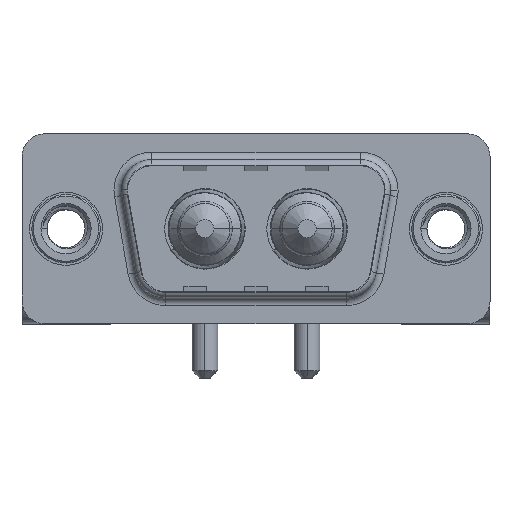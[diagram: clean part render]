
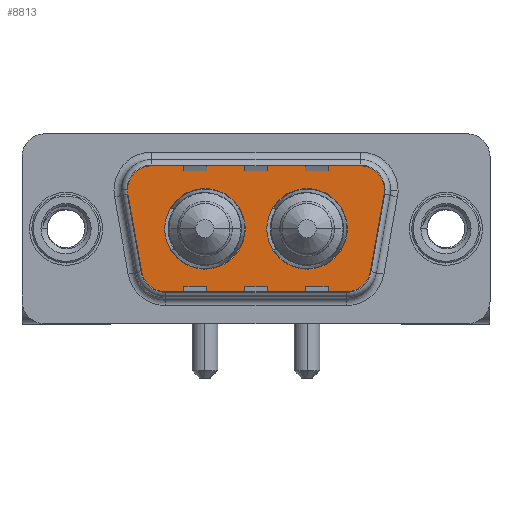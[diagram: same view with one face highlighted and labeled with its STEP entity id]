
A CAD part, top view. The second image highlights one B-rep face of the part: STEP entity #8813.
In plain terms, the highlighted planar face has unit normal (0, 0, 1).
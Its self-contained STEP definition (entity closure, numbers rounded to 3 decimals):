
#17 = LINE ( 'NONE', #8487, #10668 ) ;
#69 = VERTEX_POINT ( 'NONE', #1783 ) ;
#195 = VECTOR ( 'NONE', #10316, 1000. ) ;
#313 = ORIENTED_EDGE ( 'NONE', *, *, #13382, .T. ) ;
#531 = EDGE_CURVE ( 'NONE', #8651, #4644, #12006, .T. ) ;
#673 = AXIS2_PLACEMENT_3D ( 'NONE', #11711, #11919, #10384 ) ;
#860 = CARTESIAN_POINT ( 'NONE',  ( 15.86, 0., 0. ) ) ;
#886 = ORIENTED_EDGE ( 'NONE', *, *, #9757, .T. ) ;
#1145 = CIRCLE ( 'NONE', #2961, 2. ) ;
#1183 = CIRCLE ( 'NONE', #9352, 2.65 ) ;
#1215 = VERTEX_POINT ( 'NONE', #11139 ) ;
#1319 = ORIENTED_EDGE ( 'NONE', *, *, #2807, .F. ) ;
#1494 = AXIS2_PLACEMENT_3D ( 'NONE', #12614, #7407, #1807 ) ;
#1783 = CARTESIAN_POINT ( 'NONE',  ( 11.79, 0., 0. ) ) ;
#1807 = DIRECTION ( 'NONE',  ( 1., 0., 0. ) ) ;
#1871 = AXIS2_PLACEMENT_3D ( 'NONE', #4380, #8710, #12273 ) ;
#1963 = VECTOR ( 'NONE', #3189, 1000. ) ;
#1979 = DIRECTION ( 'NONE',  ( 0., 0., 1. ) ) ;
#2254 = EDGE_CURVE ( 'NONE', #3046, #11323, #12685, .T. ) ;
#2335 = EDGE_CURVE ( 'NONE', #69, #5789, #7602, .T. ) ;
#2347 = CARTESIAN_POINT ( 'NONE',  ( 19.564, 4.9, 0. ) ) ;
#2535 = ORIENTED_EDGE ( 'NONE', *, *, #11540, .F. ) ;
#2633 = DIRECTION ( 'NONE',  ( 0., 0., 1. ) ) ;
#2807 = EDGE_CURVE ( 'NONE', #4644, #8651, #10326, .T. ) ;
#2851 = FACE_BOUND ( 'NONE', #9070, .T. ) ;
#2918 = CARTESIAN_POINT ( 'NONE',  ( 18.541, -2.9, 0. ) ) ;
#2961 = AXIS2_PLACEMENT_3D ( 'NONE', #13447, #7103, #10376 ) ;
#3046 = VERTEX_POINT ( 'NONE', #2347 ) ;
#3189 = DIRECTION ( 'NONE',  ( 0.174, -0.985, 0. ) ) ;
#3738 = AXIS2_PLACEMENT_3D ( 'NONE', #860, #13870, #12666 ) ;
#3829 = EDGE_CURVE ( 'NONE', #12313, #10613, #10870, .T. ) ;
#3947 = CARTESIAN_POINT ( 'NONE',  ( 20.511, -3.247, 0. ) ) ;
#4380 = CARTESIAN_POINT ( 'NONE',  ( 19.564, 2.9, 0. ) ) ;
#4626 = CARTESIAN_POINT ( 'NONE',  ( 6.459, -4.9, 0. ) ) ;
#4630 = ORIENTED_EDGE ( 'NONE', *, *, #7220, .T. ) ;
#4644 = VERTEX_POINT ( 'NONE', #10782 ) ;
#4932 = DIRECTION ( 'NONE',  ( 1., 0., 0. ) ) ;
#4981 = VERTEX_POINT ( 'NONE', #11244 ) ;
#5092 = EDGE_LOOP ( 'NONE', ( #313, #8845, #9042, #886, #14020, #4630, #5809, #10586, #8516 ) ) ;
#5184 = FACE_BOUND ( 'NONE', #7694, .T. ) ;
#5206 = CIRCLE ( 'NONE', #673, 2. ) ;
#5745 = CARTESIAN_POINT ( 'NONE',  ( 6.459, -2.9, 0. ) ) ;
#5789 = VERTEX_POINT ( 'NONE', #12716 ) ;
#5809 = ORIENTED_EDGE ( 'NONE', *, *, #3829, .T. ) ;
#5972 = EDGE_CURVE ( 'NONE', #13334, #9483, #11846, .T. ) ;
#6006 = DIRECTION ( 'NONE',  ( 0., 0., 1. ) ) ;
#6139 = VERTEX_POINT ( 'NONE', #3947 ) ;
#6178 = AXIS2_PLACEMENT_3D ( 'NONE', #2918, #13797, #11588 ) ;
#7091 = EDGE_CURVE ( 'NONE', #4981, #1215, #13589, .T. ) ;
#7094 = AXIS2_PLACEMENT_3D ( 'NONE', #5745, #2633, #7872 ) ;
#7103 = DIRECTION ( 'NONE',  ( 0., 0., 1. ) ) ;
#7176 = FACE_OUTER_BOUND ( 'NONE', #5092, .T. ) ;
#7220 = EDGE_CURVE ( 'NONE', #11323, #12313, #5206, .T. ) ;
#7338 = DIRECTION ( 'NONE',  ( -1., 0., 0. ) ) ;
#7407 = DIRECTION ( 'NONE',  ( 0., 0., 1. ) ) ;
#7602 = CIRCLE ( 'NONE', #1494, 2.65 ) ;
#7645 = EDGE_CURVE ( 'NONE', #6139, #13334, #17, .T. ) ;
#7694 = EDGE_LOOP ( 'NONE', ( #7771, #2535 ) ) ;
#7771 = ORIENTED_EDGE ( 'NONE', *, *, #2335, .F. ) ;
#7872 = DIRECTION ( 'NONE',  ( -1., 0., 0. ) ) ;
#7877 = CIRCLE ( 'NONE', #13337, 2. ) ;
#8261 = ORIENTED_EDGE ( 'NONE', *, *, #531, .F. ) ;
#8487 = CARTESIAN_POINT ( 'NONE',  ( 21.534, 2.553, 0. ) ) ;
#8516 = ORIENTED_EDGE ( 'NONE', *, *, #7091, .T. ) ;
#8531 = CARTESIAN_POINT ( 'NONE',  ( 21.564, 2.9, 0. ) ) ;
#8651 = VERTEX_POINT ( 'NONE', #9173 ) ;
#8710 = DIRECTION ( 'NONE',  ( 0., 0., 1. ) ) ;
#8813 = ADVANCED_FACE ( 'NONE', ( #2851, #5184, #7176 ), #10455, .T. ) ;
#8845 = ORIENTED_EDGE ( 'NONE', *, *, #7645, .T. ) ;
#9038 = EDGE_CURVE ( 'NONE', #10613, #4981, #9348, .T. ) ;
#9042 = ORIENTED_EDGE ( 'NONE', *, *, #5972, .T. ) ;
#9070 = EDGE_LOOP ( 'NONE', ( #1319, #8261 ) ) ;
#9173 = CARTESIAN_POINT ( 'NONE',  ( 13.21, 0., 0. ) ) ;
#9348 = CIRCLE ( 'NONE', #7094, 2. ) ;
#9352 = AXIS2_PLACEMENT_3D ( 'NONE', #11413, #6006, #4932 ) ;
#9483 = VERTEX_POINT ( 'NONE', #8531 ) ;
#9757 = EDGE_CURVE ( 'NONE', #9483, #3046, #1145, .T. ) ;
#9802 = DIRECTION ( 'NONE',  ( 0., 0., 1. ) ) ;
#9943 = CARTESIAN_POINT ( 'NONE',  ( 15.86, 0., 0. ) ) ;
#10316 = DIRECTION ( 'NONE',  ( 1., 0., 0. ) ) ;
#10326 = CIRCLE ( 'NONE', #3738, 2.65 ) ;
#10371 = CARTESIAN_POINT ( 'NONE',  ( 21.534, 2.553, 0. ) ) ;
#10376 = DIRECTION ( 'NONE',  ( -1., 0., 0. ) ) ;
#10384 = DIRECTION ( 'NONE',  ( 1., 0., 0. ) ) ;
#10455 = PLANE ( 'NONE',  #6178 ) ;
#10586 = ORIENTED_EDGE ( 'NONE', *, *, #9038, .T. ) ;
#10613 = VERTEX_POINT ( 'NONE', #13670 ) ;
#10646 = DIRECTION ( 'NONE',  ( 1., 0., 0. ) ) ;
#10668 = VECTOR ( 'NONE', #13833, 1000. ) ;
#10776 = CARTESIAN_POINT ( 'NONE',  ( 5.436, 4.9, 0. ) ) ;
#10782 = CARTESIAN_POINT ( 'NONE',  ( 18.51, 0., 0. ) ) ;
#10870 = LINE ( 'NONE', #12941, #1963 ) ;
#10951 = DIRECTION ( 'NONE',  ( 1., 0., 0. ) ) ;
#11139 = CARTESIAN_POINT ( 'NONE',  ( 18.541, -4.9, 0. ) ) ;
#11244 = CARTESIAN_POINT ( 'NONE',  ( 6.459, -4.9, 0. ) ) ;
#11254 = VECTOR ( 'NONE', #7338, 1000. ) ;
#11323 = VERTEX_POINT ( 'NONE', #10776 ) ;
#11335 = AXIS2_PLACEMENT_3D ( 'NONE', #9943, #9802, #10951 ) ;
#11413 = CARTESIAN_POINT ( 'NONE',  ( 9.14, 0., 0. ) ) ;
#11540 = EDGE_CURVE ( 'NONE', #5789, #69, #1183, .T. ) ;
#11588 = DIRECTION ( 'NONE',  ( 1., 0., 0. ) ) ;
#11711 = CARTESIAN_POINT ( 'NONE',  ( 5.436, 2.9, 0. ) ) ;
#11714 = CARTESIAN_POINT ( 'NONE',  ( 18.541, -2.9, 0. ) ) ;
#11846 = CIRCLE ( 'NONE', #1871, 2. ) ;
#11919 = DIRECTION ( 'NONE',  ( 0., 0., 1. ) ) ;
#12006 = CIRCLE ( 'NONE', #11335, 2.65 ) ;
#12273 = DIRECTION ( 'NONE',  ( -1., 0., 0. ) ) ;
#12313 = VERTEX_POINT ( 'NONE', #13317 ) ;
#12614 = CARTESIAN_POINT ( 'NONE',  ( 9.14, 0., 0. ) ) ;
#12666 = DIRECTION ( 'NONE',  ( 1., 0., 0. ) ) ;
#12685 = LINE ( 'NONE', #13818, #11254 ) ;
#12716 = CARTESIAN_POINT ( 'NONE',  ( 6.49, 0., 0. ) ) ;
#12941 = CARTESIAN_POINT ( 'NONE',  ( 3.466, 2.553, 0. ) ) ;
#13317 = CARTESIAN_POINT ( 'NONE',  ( 3.466, 2.553, 0. ) ) ;
#13334 = VERTEX_POINT ( 'NONE', #10371 ) ;
#13337 = AXIS2_PLACEMENT_3D ( 'NONE', #11714, #1979, #10646 ) ;
#13382 = EDGE_CURVE ( 'NONE', #1215, #6139, #7877, .T. ) ;
#13447 = CARTESIAN_POINT ( 'NONE',  ( 19.564, 2.9, 0. ) ) ;
#13589 = LINE ( 'NONE', #4626, #195 ) ;
#13670 = CARTESIAN_POINT ( 'NONE',  ( 4.489, -3.247, 0. ) ) ;
#13797 = DIRECTION ( 'NONE',  ( 0., 0., 1. ) ) ;
#13818 = CARTESIAN_POINT ( 'NONE',  ( 5.436, 4.9, 0. ) ) ;
#13833 = DIRECTION ( 'NONE',  ( 0.174, 0.985, 0. ) ) ;
#13870 = DIRECTION ( 'NONE',  ( 0., 0., 1. ) ) ;
#14020 = ORIENTED_EDGE ( 'NONE', *, *, #2254, .T. ) ;
